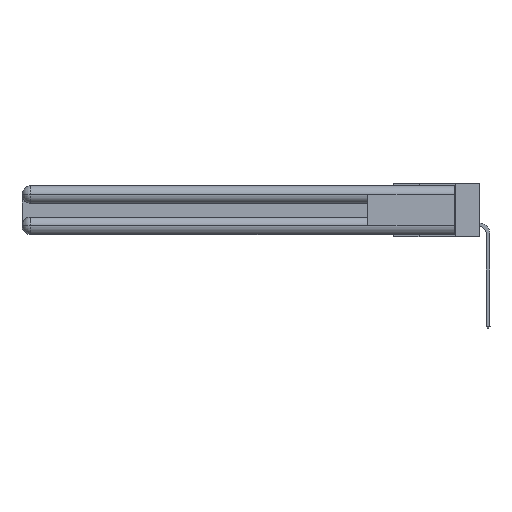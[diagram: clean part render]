
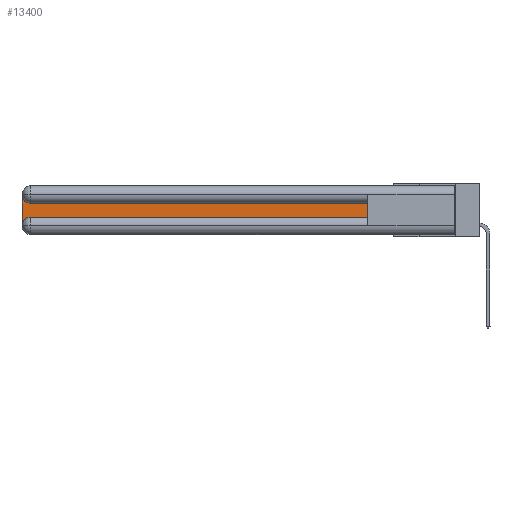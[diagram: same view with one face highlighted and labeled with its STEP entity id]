
A CAD part, left-side view. The second image highlights one B-rep face of the part: STEP entity #13400.
In plain terms, the highlighted planar face has unit normal (-1, 0, 0).
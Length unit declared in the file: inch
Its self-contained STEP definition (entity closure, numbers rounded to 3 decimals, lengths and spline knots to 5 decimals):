
#2229 = CARTESIAN_POINT ( 'NONE',  ( 0.075, 2.94, -0.1225 ) ) ;
#2798 = VERTEX_POINT ( 'NONE', #2916 ) ;
#2916 = CARTESIAN_POINT ( 'NONE',  ( 0.075, 0.6, -0.2175 ) ) ;
#3320 = DIRECTION ( 'NONE',  ( 0., 0., 1. ) ) ;
#3412 = LINE ( 'NONE', #8584, #17533 ) ;
#4185 = VECTOR ( 'NONE', #3320, 39.37008 ) ;
#5803 = DIRECTION ( 'NONE',  ( 0., 0., -1. ) ) ;
#5840 = AXIS2_PLACEMENT_3D ( 'NONE', #6465, #24591, #26861 ) ;
#6242 = ORIENTED_EDGE ( 'NONE', *, *, #17056, .T. ) ;
#6465 = CARTESIAN_POINT ( 'NONE',  ( 0.075, 2.94, -0.0625 ) ) ;
#6681 = VERTEX_POINT ( 'NONE', #9640 ) ;
#7058 = VERTEX_POINT ( 'NONE', #2229 ) ;
#7251 = CARTESIAN_POINT ( 'NONE',  ( 0.075, 3., -0.2775 ) ) ;
#7530 = VECTOR ( 'NONE', #9978, 39.37008 ) ;
#7689 = CARTESIAN_POINT ( 'NONE',  ( 0.075, 2.94, -0.2175 ) ) ;
#7787 = CARTESIAN_POINT ( 'NONE',  ( 0.075, 3., -0.1225 ) ) ;
#8533 = EDGE_CURVE ( 'NONE', #6681, #18841, #23427, .T. ) ;
#8584 = CARTESIAN_POINT ( 'NONE',  ( 0.075, 0.6, -0.1225 ) ) ;
#8670 = EDGE_CURVE ( 'NONE', #26559, #2798, #18154, .T. ) ;
#9640 = CARTESIAN_POINT ( 'NONE',  ( 0.075, 3., -0.0625 ) ) ;
#9720 = CIRCLE ( 'NONE', #19213, 0.06 ) ;
#9978 = DIRECTION ( 'NONE',  ( 0., 0., -1. ) ) ;
#10363 = VERTEX_POINT ( 'NONE', #26830 ) ;
#10518 = ORIENTED_EDGE ( 'NONE', *, *, #8670, .T. ) ;
#12588 = CARTESIAN_POINT ( 'NONE',  ( 0.075, 0.6, -0.2175 ) ) ;
#13021 = EDGE_LOOP ( 'NONE', ( #18682, #19334, #29186, #6242, #10518, #22708 ) ) ;
#13400 = ADVANCED_FACE ( 'NONE', ( #20798 ), #14622, .F. ) ;
#14447 = CARTESIAN_POINT ( 'NONE',  ( 0.075, 3., -0.2175 ) ) ;
#14622 = PLANE ( 'NONE',  #15214 ) ;
#15214 = AXIS2_PLACEMENT_3D ( 'NONE', #7787, #21383, #5803 ) ;
#15368 = DIRECTION ( 'NONE',  ( 0., 0., -1. ) ) ;
#17056 = EDGE_CURVE ( 'NONE', #18841, #26559, #9720, .T. ) ;
#17533 = VECTOR ( 'NONE', #21966, 39.37008 ) ;
#18154 = LINE ( 'NONE', #23944, #24109 ) ;
#18682 = ORIENTED_EDGE ( 'NONE', *, *, #23640, .T. ) ;
#18841 = VERTEX_POINT ( 'NONE', #7251 ) ;
#19213 = AXIS2_PLACEMENT_3D ( 'NONE', #23321, #19991, #15368 ) ;
#19334 = ORIENTED_EDGE ( 'NONE', *, *, #21305, .T. ) ;
#19404 = CIRCLE ( 'NONE', #5840, 0.06 ) ;
#19991 = DIRECTION ( 'NONE',  ( 1., 0., 0. ) ) ;
#20798 = FACE_OUTER_BOUND ( 'NONE', #13021, .T. ) ;
#21305 = EDGE_CURVE ( 'NONE', #7058, #6681, #19404, .T. ) ;
#21383 = DIRECTION ( 'NONE',  ( 1., 0., 0. ) ) ;
#21509 = DIRECTION ( 'NONE',  ( 0., -1., 0. ) ) ;
#21737 = EDGE_CURVE ( 'NONE', #2798, #10363, #29178, .T. ) ;
#21966 = DIRECTION ( 'NONE',  ( 0., 1., 0. ) ) ;
#22708 = ORIENTED_EDGE ( 'NONE', *, *, #21737, .T. ) ;
#23321 = CARTESIAN_POINT ( 'NONE',  ( 0.075, 2.94, -0.2775 ) ) ;
#23427 = LINE ( 'NONE', #14447, #7530 ) ;
#23640 = EDGE_CURVE ( 'NONE', #10363, #7058, #3412, .T. ) ;
#23944 = CARTESIAN_POINT ( 'NONE',  ( 0.075, 0.6, -0.2175 ) ) ;
#24109 = VECTOR ( 'NONE', #21509, 39.37008 ) ;
#24591 = DIRECTION ( 'NONE',  ( 1., 0., 0. ) ) ;
#26559 = VERTEX_POINT ( 'NONE', #7689 ) ;
#26830 = CARTESIAN_POINT ( 'NONE',  ( 0.075, 0.6, -0.1225 ) ) ;
#26861 = DIRECTION ( 'NONE',  ( 0., 0., -1. ) ) ;
#29178 = LINE ( 'NONE', #12588, #4185 ) ;
#29186 = ORIENTED_EDGE ( 'NONE', *, *, #8533, .T. ) ;
